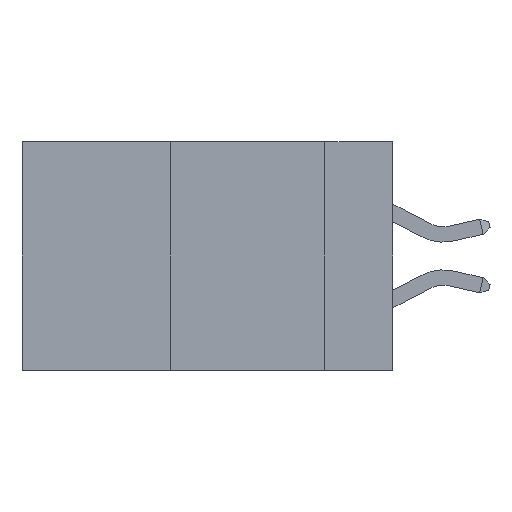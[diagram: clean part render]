
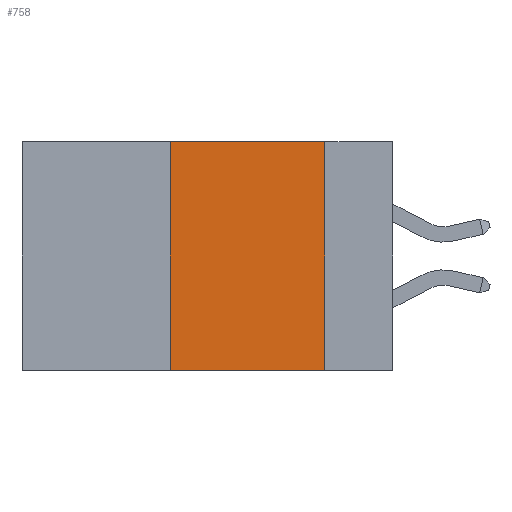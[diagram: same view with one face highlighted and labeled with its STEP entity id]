
A CAD part, left-side view. The second image highlights one B-rep face of the part: STEP entity #758.
In plain terms, the highlighted planar face has unit normal (-1, 0, 0).
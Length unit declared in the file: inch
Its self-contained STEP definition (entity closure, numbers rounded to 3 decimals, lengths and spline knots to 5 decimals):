
#758 = ADVANCED_FACE ( 'NONE', ( #12045 ), #15741, .F. ) ;
#1318 = ORIENTED_EDGE ( 'NONE', *, *, #9821, .T. ) ;
#1892 = CARTESIAN_POINT ( 'NONE',  ( 0., 0.11, 0. ) ) ;
#2903 = VERTEX_POINT ( 'NONE', #9854 ) ;
#3685 = DIRECTION ( 'NONE',  ( 0., -1., 0. ) ) ;
#4836 = EDGE_LOOP ( 'NONE', ( #7141, #13877, #5337, #1318 ) ) ;
#5201 = VECTOR ( 'NONE', #8479, 39.37008 ) ;
#5337 = ORIENTED_EDGE ( 'NONE', *, *, #7927, .F. ) ;
#6782 = LINE ( 'NONE', #15813, #12519 ) ;
#7141 = ORIENTED_EDGE ( 'NONE', *, *, #9559, .F. ) ;
#7285 = CARTESIAN_POINT ( 'NONE',  ( 0., 0.36, -0.37 ) ) ;
#7526 = DIRECTION ( 'NONE',  ( 0., 0., 1. ) ) ;
#7597 = DIRECTION ( 'NONE',  ( 0., -1., 0. ) ) ;
#7927 = EDGE_CURVE ( 'NONE', #9924, #15086, #6782, .T. ) ;
#8349 = CARTESIAN_POINT ( 'NONE',  ( 0., 0.11, 0. ) ) ;
#8479 = DIRECTION ( 'NONE',  ( 0., 0., -1. ) ) ;
#9482 = LINE ( 'NONE', #15566, #9685 ) ;
#9559 = EDGE_CURVE ( 'NONE', #11115, #2903, #12843, .T. ) ;
#9685 = VECTOR ( 'NONE', #7597, 39.37008 ) ;
#9821 = EDGE_CURVE ( 'NONE', #9924, #2903, #9482, .T. ) ;
#9854 = CARTESIAN_POINT ( 'NONE',  ( 0., 0.11, -0.37 ) ) ;
#9924 = VERTEX_POINT ( 'NONE', #7285 ) ;
#10365 = DIRECTION ( 'NONE',  ( 1., 0., 0. ) ) ;
#10387 = VECTOR ( 'NONE', #3685, 39.37008 ) ;
#11115 = VERTEX_POINT ( 'NONE', #1892 ) ;
#11560 = CARTESIAN_POINT ( 'NONE',  ( 0., 0.6, 0. ) ) ;
#12045 = FACE_OUTER_BOUND ( 'NONE', #4836, .T. ) ;
#12519 = VECTOR ( 'NONE', #7526, 39.37008 ) ;
#12843 = LINE ( 'NONE', #8349, #5201 ) ;
#12974 = EDGE_CURVE ( 'NONE', #15086, #11115, #14306, .T. ) ;
#13561 = DIRECTION ( 'NONE',  ( 0., 0., -1. ) ) ;
#13645 = CARTESIAN_POINT ( 'NONE',  ( 0., 0.6, 0. ) ) ;
#13877 = ORIENTED_EDGE ( 'NONE', *, *, #12974, .F. ) ;
#14306 = LINE ( 'NONE', #11560, #10387 ) ;
#14571 = AXIS2_PLACEMENT_3D ( 'NONE', #13645, #10365, #13561 ) ;
#14625 = CARTESIAN_POINT ( 'NONE',  ( 0., 0.36, 0. ) ) ;
#15086 = VERTEX_POINT ( 'NONE', #14625 ) ;
#15566 = CARTESIAN_POINT ( 'NONE',  ( 0., 0.6, -0.37 ) ) ;
#15741 = PLANE ( 'NONE',  #14571 ) ;
#15813 = CARTESIAN_POINT ( 'NONE',  ( 0., 0.36, 0. ) ) ;
